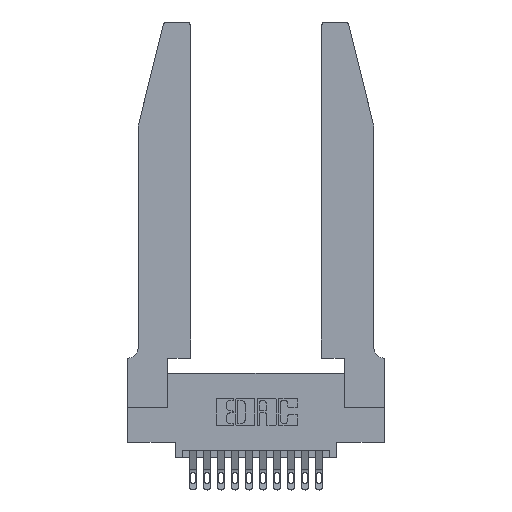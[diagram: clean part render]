
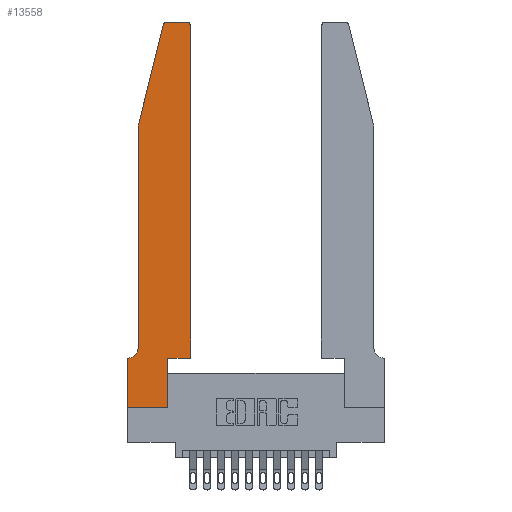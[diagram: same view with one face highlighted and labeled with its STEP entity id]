
A CAD part, top view. The second image highlights one B-rep face of the part: STEP entity #13558.
In plain terms, the highlighted planar face has unit normal (0, 0, 1).
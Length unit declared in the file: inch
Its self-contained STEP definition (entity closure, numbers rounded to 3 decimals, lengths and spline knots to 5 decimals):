
#448 = EDGE_CURVE ( 'NONE', #5627, #15730, #1987, .T. ) ;
#511 = DIRECTION ( 'NONE',  ( 0., 0., -1. ) ) ;
#575 = ORIENTED_EDGE ( 'NONE', *, *, #7251, .T. ) ;
#1076 = ORIENTED_EDGE ( 'NONE', *, *, #5475, .T. ) ;
#1524 = VECTOR ( 'NONE', #11662, 39.37008 ) ;
#1551 = CARTESIAN_POINT ( 'NONE',  ( 0.25487, 2.72718, 0.37 ) ) ;
#1987 = LINE ( 'NONE', #16867, #1524 ) ;
#2094 = LINE ( 'NONE', #16856, #14972 ) ;
#2101 = DIRECTION ( 'NONE',  ( -1., 0., 0. ) ) ;
#2373 = VERTEX_POINT ( 'NONE', #4621 ) ;
#2381 = DIRECTION ( 'NONE',  ( 0., 0., 1. ) ) ;
#2618 = ORIENTED_EDGE ( 'NONE', *, *, #15861, .T. ) ;
#2753 = VERTEX_POINT ( 'NONE', #4376 ) ;
#2808 = EDGE_CURVE ( 'NONE', #9249, #15723, #2094, .T. ) ;
#2993 = ORIENTED_EDGE ( 'NONE', *, *, #2808, .T. ) ;
#3133 = ORIENTED_EDGE ( 'NONE', *, *, #15470, .T. ) ;
#3184 = DIRECTION ( 'NONE',  ( 0., 0., 1. ) ) ;
#3351 = VERTEX_POINT ( 'NONE', #11102 ) ;
#3356 = EDGE_CURVE ( 'NONE', #3427, #2373, #8799, .T. ) ;
#3427 = VERTEX_POINT ( 'NONE', #6462 ) ;
#3468 = ORIENTED_EDGE ( 'NONE', *, *, #3510, .T. ) ;
#3472 = ORIENTED_EDGE ( 'NONE', *, *, #3356, .T. ) ;
#3510 = EDGE_CURVE ( 'NONE', #4719, #2753, #12894, .T. ) ;
#3750 = FACE_OUTER_BOUND ( 'NONE', #6098, .T. ) ;
#4376 = CARTESIAN_POINT ( 'NONE',  ( 0., 0., 0.37 ) ) ;
#4621 = CARTESIAN_POINT ( 'NONE',  ( 0.4505, 2.72, 0.37 ) ) ;
#4719 = VERTEX_POINT ( 'NONE', #12855 ) ;
#4792 = CARTESIAN_POINT ( 'NONE',  ( 0.0755, 2., 0.37 ) ) ;
#4991 = AXIS2_PLACEMENT_3D ( 'NONE', #8703, #511, #10031 ) ;
#5282 = VECTOR ( 'NONE', #11042, 39.37008 ) ;
#5431 = CIRCLE ( 'NONE', #11006, 0.03 ) ;
#5448 = VERTEX_POINT ( 'NONE', #13823 ) ;
#5453 = CARTESIAN_POINT ( 'NONE',  ( 0.4205, 2.72, 0.37 ) ) ;
#5475 = EDGE_CURVE ( 'NONE', #15730, #3427, #12646, .T. ) ;
#5627 = VERTEX_POINT ( 'NONE', #10269 ) ;
#5962 = VECTOR ( 'NONE', #11137, 39.37008 ) ;
#6062 = DIRECTION ( 'NONE',  ( 1., 0., 0. ) ) ;
#6098 = EDGE_LOOP ( 'NONE', ( #2618, #15280, #2993, #575, #3133, #7832, #3468, #10848, #10448, #1076, #3472, #14605 ) ) ;
#6462 = CARTESIAN_POINT ( 'NONE',  ( 0.4505, 0.35, 0.37 ) ) ;
#6586 = CARTESIAN_POINT ( 'NONE',  ( 0.2865, 0.35, 0.37 ) ) ;
#6770 = DIRECTION ( 'NONE',  ( 1., 0., 0. ) ) ;
#7122 = VECTOR ( 'NONE', #12131, 39.37008 ) ;
#7251 = EDGE_CURVE ( 'NONE', #15723, #8176, #10755, .T. ) ;
#7271 = VECTOR ( 'NONE', #13882, 39.37008 ) ;
#7516 = LINE ( 'NONE', #9487, #7122 ) ;
#7832 = ORIENTED_EDGE ( 'NONE', *, *, #12939, .T. ) ;
#7973 = VECTOR ( 'NONE', #10001, 39.37008 ) ;
#8176 = VERTEX_POINT ( 'NONE', #15859 ) ;
#8703 = CARTESIAN_POINT ( 'NONE',  ( 0.0055, 0.42, 0.37 ) ) ;
#8746 = LINE ( 'NONE', #14927, #5282 ) ;
#8799 = LINE ( 'NONE', #14664, #7973 ) ;
#9164 = VECTOR ( 'NONE', #6062, 39.37008 ) ;
#9209 = CARTESIAN_POINT ( 'NONE',  ( 0.0755, 2., 0.37 ) ) ;
#9249 = VERTEX_POINT ( 'NONE', #1551 ) ;
#9421 = CARTESIAN_POINT ( 'NONE',  ( 0., 0., 0.37 ) ) ;
#9487 = CARTESIAN_POINT ( 'NONE',  ( 0.2605, 2.75, 0.37 ) ) ;
#9561 = CIRCLE ( 'NONE', #12534, 0.03 ) ;
#10001 = DIRECTION ( 'NONE',  ( 0., 1., 0. ) ) ;
#10031 = DIRECTION ( 'NONE',  ( -1., 0., 0. ) ) ;
#10269 = CARTESIAN_POINT ( 'NONE',  ( 0.2865, 0., 0.37 ) ) ;
#10384 = CARTESIAN_POINT ( 'NONE',  ( 0., 0.35, 0.37 ) ) ;
#10448 = ORIENTED_EDGE ( 'NONE', *, *, #448, .T. ) ;
#10755 = LINE ( 'NONE', #4792, #7271 ) ;
#10848 = ORIENTED_EDGE ( 'NONE', *, *, #12210, .T. ) ;
#11006 = AXIS2_PLACEMENT_3D ( 'NONE', #11126, #3184, #12422 ) ;
#11042 = DIRECTION ( 'NONE',  ( 1., 0., 0. ) ) ;
#11102 = CARTESIAN_POINT ( 'NONE',  ( 0.0055, 0.35, 0.37 ) ) ;
#11126 = CARTESIAN_POINT ( 'NONE',  ( 0.284, 2.72, 0.37 ) ) ;
#11137 = DIRECTION ( 'NONE',  ( 0., -1., 0. ) ) ;
#11645 = PLANE ( 'NONE',  #13950 ) ;
#11662 = DIRECTION ( 'NONE',  ( 0., 1., 0. ) ) ;
#11701 = DIRECTION ( 'NONE',  ( 1., 0., 0. ) ) ;
#12006 = VECTOR ( 'NONE', #2101, 39.37008 ) ;
#12131 = DIRECTION ( 'NONE',  ( -1., 0., 0. ) ) ;
#12210 = EDGE_CURVE ( 'NONE', #2753, #5627, #8746, .T. ) ;
#12422 = DIRECTION ( 'NONE',  ( 1., 0., 0. ) ) ;
#12534 = AXIS2_PLACEMENT_3D ( 'NONE', #5453, #14593, #6770 ) ;
#12646 = LINE ( 'NONE', #13877, #9164 ) ;
#12749 = VERTEX_POINT ( 'NONE', #13265 ) ;
#12767 = DIRECTION ( 'NONE',  ( -0.239, -0.971, 0. ) ) ;
#12855 = CARTESIAN_POINT ( 'NONE',  ( 0., 0.35, 0.37 ) ) ;
#12894 = LINE ( 'NONE', #9421, #5962 ) ;
#12939 = EDGE_CURVE ( 'NONE', #3351, #4719, #15505, .T. ) ;
#13265 = CARTESIAN_POINT ( 'NONE',  ( 0.4205, 2.75, 0.37 ) ) ;
#13558 = ADVANCED_FACE ( 'NONE', ( #3750 ), #11645, .T. ) ;
#13687 = CIRCLE ( 'NONE', #4991, 0.07 ) ;
#13823 = CARTESIAN_POINT ( 'NONE',  ( 0.284, 2.75, 0.37 ) ) ;
#13877 = CARTESIAN_POINT ( 'NONE',  ( 0.4505, 0.35, 0.37 ) ) ;
#13882 = DIRECTION ( 'NONE',  ( 0., -1., 0. ) ) ;
#13925 = EDGE_CURVE ( 'NONE', #5448, #9249, #5431, .T. ) ;
#13950 = AXIS2_PLACEMENT_3D ( 'NONE', #10384, #2381, #11701 ) ;
#14593 = DIRECTION ( 'NONE',  ( 0., 0., 1. ) ) ;
#14605 = ORIENTED_EDGE ( 'NONE', *, *, #15785, .T. ) ;
#14664 = CARTESIAN_POINT ( 'NONE',  ( 0.4505, 0.35, 0.37 ) ) ;
#14927 = CARTESIAN_POINT ( 'NONE',  ( 0., 0., 0.37 ) ) ;
#14972 = VECTOR ( 'NONE', #12767, 39.37008 ) ;
#15280 = ORIENTED_EDGE ( 'NONE', *, *, #13925, .T. ) ;
#15355 = CARTESIAN_POINT ( 'NONE',  ( 0.0755, 0.35, 0.37 ) ) ;
#15470 = EDGE_CURVE ( 'NONE', #8176, #3351, #13687, .T. ) ;
#15505 = LINE ( 'NONE', #15355, #12006 ) ;
#15723 = VERTEX_POINT ( 'NONE', #9209 ) ;
#15730 = VERTEX_POINT ( 'NONE', #6586 ) ;
#15785 = EDGE_CURVE ( 'NONE', #2373, #12749, #9561, .T. ) ;
#15859 = CARTESIAN_POINT ( 'NONE',  ( 0.0755, 0.42, 0.37 ) ) ;
#15861 = EDGE_CURVE ( 'NONE', #12749, #5448, #7516, .T. ) ;
#16856 = CARTESIAN_POINT ( 'NONE',  ( 0.0755, 2., 0.37 ) ) ;
#16867 = CARTESIAN_POINT ( 'NONE',  ( 0.2865, 0.35, 0.37 ) ) ;
